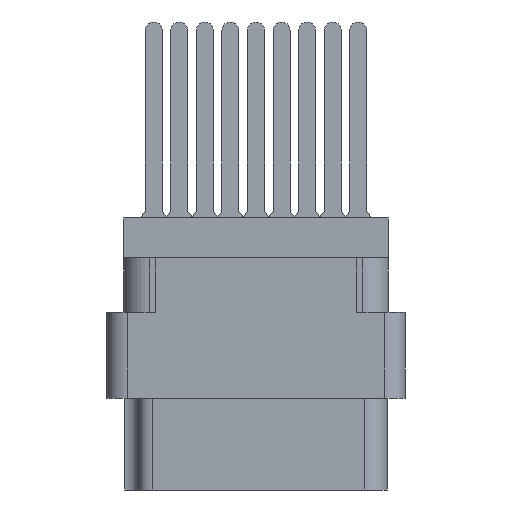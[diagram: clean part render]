
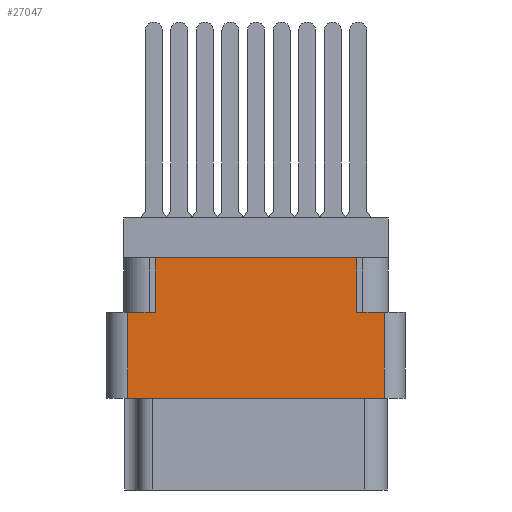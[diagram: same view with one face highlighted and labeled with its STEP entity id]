
A CAD part, left-side view. The second image highlights one B-rep face of the part: STEP entity #27047.
In plain terms, the highlighted planar face has unit normal (-1, 0, 0).
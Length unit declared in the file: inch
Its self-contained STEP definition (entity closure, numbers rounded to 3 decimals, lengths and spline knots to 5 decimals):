
#1372 = CARTESIAN_POINT ( 'NONE',  ( -1.296, -0.438, -0.798 ) ) ;
#1405 = DIRECTION ( 'NONE',  ( 0., 0., 1. ) ) ;
#1522 = PLANE ( 'NONE',  #17573 ) ;
#1714 = EDGE_CURVE ( 'NONE', #12007, #6219, #25600, .T. ) ;
#1816 = DIRECTION ( 'NONE',  ( 0., 0., 1. ) ) ;
#4138 = ORIENTED_EDGE ( 'NONE', *, *, #27050, .F. ) ;
#4569 = VECTOR ( 'NONE', #21507, 39.37008 ) ;
#5359 = DIRECTION ( 'NONE',  ( 0., -1., 0. ) ) ;
#5574 = CARTESIAN_POINT ( 'NONE',  ( -1.296, 0., -0.277 ) ) ;
#5712 = LINE ( 'NONE', #32280, #4569 ) ;
#6219 = VERTEX_POINT ( 'NONE', #41475 ) ;
#6228 = ORIENTED_EDGE ( 'NONE', *, *, #6314, .T. ) ;
#6314 = EDGE_CURVE ( 'NONE', #12007, #12878, #19999, .T. ) ;
#7255 = LINE ( 'NONE', #34253, #20324 ) ;
#7261 = CARTESIAN_POINT ( 'NONE',  ( -1.296, 0.438, -0.117 ) ) ;
#7399 = DIRECTION ( 'NONE',  ( 0., 0., 1. ) ) ;
#8584 = VERTEX_POINT ( 'NONE', #38578 ) ;
#8693 = DIRECTION ( 'NONE',  ( 0., 0., 1. ) ) ;
#9196 = CARTESIAN_POINT ( 'NONE',  ( -1.296, -0.376, -0.798 ) ) ;
#10089 = DIRECTION ( 'NONE',  ( 0., -1., 0. ) ) ;
#10420 = EDGE_LOOP ( 'NONE', ( #4138, #19005, #12724, #20417, #13997, #6228, #17620, #11794 ) ) ;
#10538 = EDGE_CURVE ( 'NONE', #46343, #27369, #23782, .T. ) ;
#10648 = LINE ( 'NONE', #36017, #24902 ) ;
#11230 = EDGE_CURVE ( 'NONE', #19009, #12878, #28857, .T. ) ;
#11794 = ORIENTED_EDGE ( 'NONE', *, *, #15919, .F. ) ;
#12007 = VERTEX_POINT ( 'NONE', #16405 ) ;
#12162 = VECTOR ( 'NONE', #1405, 39.37008 ) ;
#12724 = ORIENTED_EDGE ( 'NONE', *, *, #10538, .F. ) ;
#12878 = VERTEX_POINT ( 'NONE', #29696 ) ;
#13634 = VECTOR ( 'NONE', #41870, 39.37008 ) ;
#13997 = ORIENTED_EDGE ( 'NONE', *, *, #1714, .F. ) ;
#14043 = VECTOR ( 'NONE', #46391, 39.37008 ) ;
#15919 = EDGE_CURVE ( 'NONE', #8584, #19009, #10648, .T. ) ;
#16405 = CARTESIAN_POINT ( 'NONE',  ( -1.296, -0.296, -0.277 ) ) ;
#17573 = AXIS2_PLACEMENT_3D ( 'NONE', #1372, #30469, #8693 ) ;
#17620 = ORIENTED_EDGE ( 'NONE', *, *, #11230, .F. ) ;
#18830 = EDGE_CURVE ( 'NONE', #46343, #6219, #30374, .T. ) ;
#19005 = ORIENTED_EDGE ( 'NONE', *, *, #24569, .T. ) ;
#19009 = VERTEX_POINT ( 'NONE', #20676 ) ;
#19304 = CARTESIAN_POINT ( 'NONE',  ( -1.296, 0.376, -0.529 ) ) ;
#19999 = LINE ( 'NONE', #31075, #45120 ) ;
#20324 = VECTOR ( 'NONE', #5359, 39.37008 ) ;
#20417 = ORIENTED_EDGE ( 'NONE', *, *, #18830, .T. ) ;
#20676 = CARTESIAN_POINT ( 'NONE',  ( -1.296, 0.296, -0.117 ) ) ;
#20857 = FACE_OUTER_BOUND ( 'NONE', #10420, .T. ) ;
#21507 = DIRECTION ( 'NONE',  ( 0., 0., -1. ) ) ;
#23782 = LINE ( 'NONE', #36159, #14043 ) ;
#24569 = EDGE_CURVE ( 'NONE', #29664, #27369, #5712, .T. ) ;
#24902 = VECTOR ( 'NONE', #7399, 39.37008 ) ;
#25600 = LINE ( 'NONE', #5574, #13634 ) ;
#26506 = CARTESIAN_POINT ( 'NONE',  ( -1.296, -0.376, -0.529 ) ) ;
#27047 = ADVANCED_FACE ( 'NONE', ( #20857 ), #1522, .T. ) ;
#27050 = EDGE_CURVE ( 'NONE', #29664, #8584, #7255, .T. ) ;
#27369 = VERTEX_POINT ( 'NONE', #19304 ) ;
#28857 = LINE ( 'NONE', #7261, #37376 ) ;
#29664 = VERTEX_POINT ( 'NONE', #42039 ) ;
#29696 = CARTESIAN_POINT ( 'NONE',  ( -1.296, -0.296, -0.117 ) ) ;
#30374 = LINE ( 'NONE', #9196, #12162 ) ;
#30469 = DIRECTION ( 'NONE',  ( -1., 0., 0. ) ) ;
#31075 = CARTESIAN_POINT ( 'NONE',  ( -1.296, -0.296, -0.277 ) ) ;
#32280 = CARTESIAN_POINT ( 'NONE',  ( -1.296, 0.376, -0.798 ) ) ;
#34253 = CARTESIAN_POINT ( 'NONE',  ( -1.296, 0., -0.277 ) ) ;
#36017 = CARTESIAN_POINT ( 'NONE',  ( -1.296, 0.296, -0.277 ) ) ;
#36159 = CARTESIAN_POINT ( 'NONE',  ( -1.296, 0., -0.529 ) ) ;
#37376 = VECTOR ( 'NONE', #10089, 39.37008 ) ;
#38578 = CARTESIAN_POINT ( 'NONE',  ( -1.296, 0.296, -0.277 ) ) ;
#41475 = CARTESIAN_POINT ( 'NONE',  ( -1.296, -0.376, -0.277 ) ) ;
#41870 = DIRECTION ( 'NONE',  ( 0., -1., 0. ) ) ;
#42039 = CARTESIAN_POINT ( 'NONE',  ( -1.296, 0.376, -0.277 ) ) ;
#45120 = VECTOR ( 'NONE', #1816, 39.37008 ) ;
#46343 = VERTEX_POINT ( 'NONE', #26506 ) ;
#46391 = DIRECTION ( 'NONE',  ( 0., 1., 0. ) ) ;
